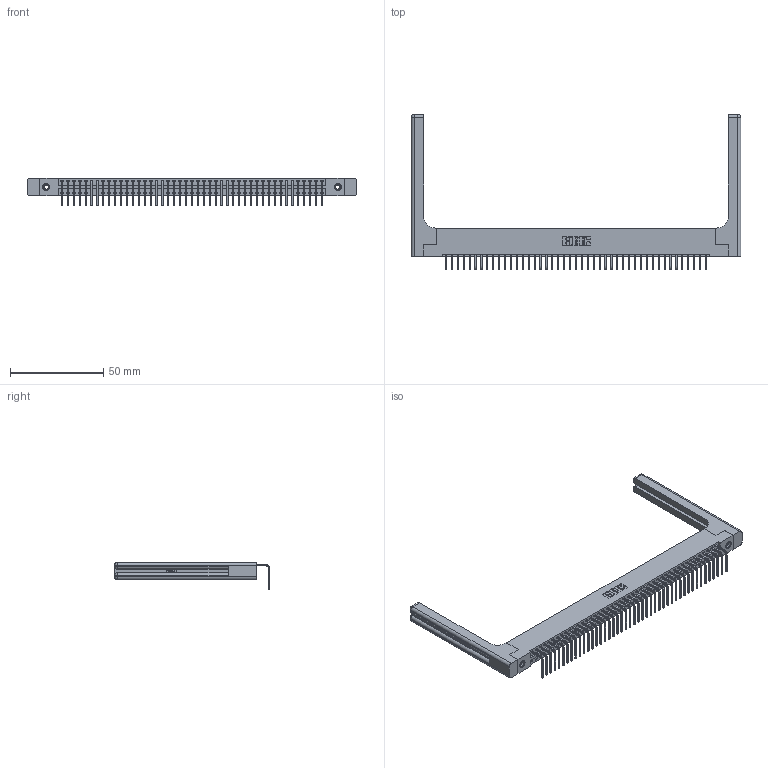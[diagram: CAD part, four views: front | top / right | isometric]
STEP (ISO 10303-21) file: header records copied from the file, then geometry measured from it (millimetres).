
FILE_DESCRIPTION (( 'STEP AP203' ), '1' );
FILE_NAME ('396-045-558-158.STEP', '2019-11-01T08:12:28', ( '' ), ( '' ), 'SwSTEP 2.0', 'SolidWorks 2016', '' );
FILE_SCHEMA (( 'CONFIG_CONTROL_DESIGN' ));
Length unit declared in the file: inch
Products named in the file (5): 396-045-558-158; 346 Part_Flush Mounting Lugs - 0.156 Dia-TH; 345-292-001_558 Tail - 2; 345-250-001_345-250-001-102; 346-220-058_345-220-058
Assembly tree (50 placements, depth 2):
  396-045-558-158
    346 Part_Flush Mounting Lugs - 0.156 Dia-TH
    345-292-001_558 Tail - 2  x45
    345-250-001_345-250-001-102  x2
    346-220-058_345-220-058  x2
Bounding box: 176.94 x 83.12 x 14.73 mm (x, y, z)
Volume: 24625.7 mm3; surface area: 27478.3 mm2
Topology: 50 solids, 50 shells, 3078 faces, 9185 edges, 6042 vertices
Faces by surface type: plane 2114, cylinder 904, bspline 36, cone 12, sphere 8, torus 4
Entity records: 32790 total; most frequent: CARTESIAN_POINT 6600, ORIENTED_EDGE 5376, DIRECTION 4750, EDGE_CURVE 2688, VECTOR 2284, LINE 2284, VERTEX_POINT 1782, AXIS2_PLACEMENT_3D 1233
